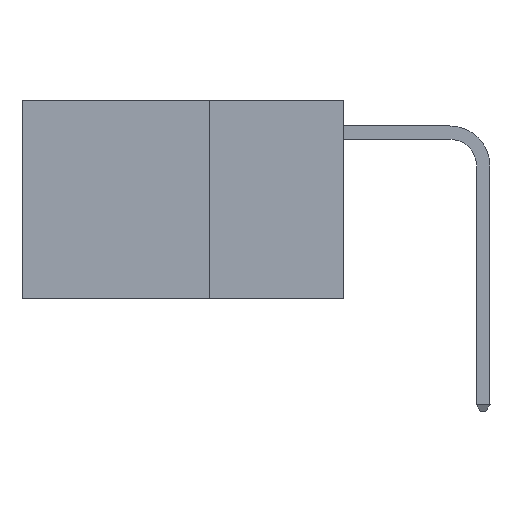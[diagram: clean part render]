
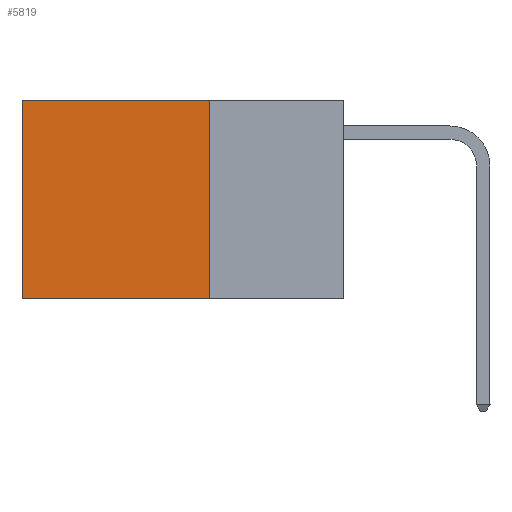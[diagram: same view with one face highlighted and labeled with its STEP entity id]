
A CAD part, left-side view. The second image highlights one B-rep face of the part: STEP entity #5819.
In plain terms, the highlighted planar face has unit normal (-1, 0, 0).
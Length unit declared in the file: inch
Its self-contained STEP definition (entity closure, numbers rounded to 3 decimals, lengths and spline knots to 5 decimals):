
#1422 = DIRECTION ( 'NONE',  ( 0., 0., -1. ) ) ;
#1533 = CARTESIAN_POINT ( 'NONE',  ( 0.2625, 0.25, 0. ) ) ;
#1546 = CARTESIAN_POINT ( 'NONE',  ( 0.2625, 0.6, 0. ) ) ;
#2012 = ORIENTED_EDGE ( 'NONE', *, *, #9931, .F. ) ;
#2030 = VERTEX_POINT ( 'NONE', #15857 ) ;
#3189 = FACE_OUTER_BOUND ( 'NONE', #8906, .T. ) ;
#3850 = VERTEX_POINT ( 'NONE', #1533 ) ;
#4911 = DIRECTION ( 'NONE',  ( 0., 0., -1. ) ) ;
#5016 = CARTESIAN_POINT ( 'NONE',  ( 0.2625, 0.25, 0. ) ) ;
#5265 = DIRECTION ( 'NONE',  ( 0., 1., 0. ) ) ;
#5454 = CARTESIAN_POINT ( 'NONE',  ( 0.2625, 0.25, 0. ) ) ;
#5637 = VECTOR ( 'NONE', #6112, 39.37008 ) ;
#5819 = ADVANCED_FACE ( 'NONE', ( #3189 ), #13883, .F. ) ;
#6083 = LINE ( 'NONE', #1546, #6202 ) ;
#6112 = DIRECTION ( 'NONE',  ( 0., 1., 0. ) ) ;
#6154 = VERTEX_POINT ( 'NONE', #17012 ) ;
#6202 = VECTOR ( 'NONE', #1422, 39.37008 ) ;
#6820 = ORIENTED_EDGE ( 'NONE', *, *, #7748, .T. ) ;
#7059 = ORIENTED_EDGE ( 'NONE', *, *, #8143, .T. ) ;
#7748 = EDGE_CURVE ( 'NONE', #3850, #2030, #8345, .T. ) ;
#7772 = EDGE_CURVE ( 'NONE', #3850, #8298, #8010, .T. ) ;
#7924 = VECTOR ( 'NONE', #4911, 39.37008 ) ;
#7942 = CARTESIAN_POINT ( 'NONE',  ( 0.2625, 0.25, -0.37 ) ) ;
#8010 = LINE ( 'NONE', #5016, #7924 ) ;
#8143 = EDGE_CURVE ( 'NONE', #2030, #6154, #6083, .T. ) ;
#8298 = VERTEX_POINT ( 'NONE', #7942 ) ;
#8345 = LINE ( 'NONE', #5454, #8379 ) ;
#8379 = VECTOR ( 'NONE', #5265, 39.37008 ) ;
#8906 = EDGE_LOOP ( 'NONE', ( #7059, #2012, #17795, #6820 ) ) ;
#9931 = EDGE_CURVE ( 'NONE', #8298, #6154, #12962, .T. ) ;
#12689 = CARTESIAN_POINT ( 'NONE',  ( 0.2625, 0.25, 0. ) ) ;
#12962 = LINE ( 'NONE', #15616, #5637 ) ;
#13620 = AXIS2_PLACEMENT_3D ( 'NONE', #12689, #17352, #17408 ) ;
#13883 = PLANE ( 'NONE',  #13620 ) ;
#15616 = CARTESIAN_POINT ( 'NONE',  ( 0.2625, 0.25, -0.37 ) ) ;
#15857 = CARTESIAN_POINT ( 'NONE',  ( 0.2625, 0.6, 0. ) ) ;
#17012 = CARTESIAN_POINT ( 'NONE',  ( 0.2625, 0.6, -0.37 ) ) ;
#17352 = DIRECTION ( 'NONE',  ( 1., 0., 0. ) ) ;
#17408 = DIRECTION ( 'NONE',  ( 0., 0., -1. ) ) ;
#17795 = ORIENTED_EDGE ( 'NONE', *, *, #7772, .F. ) ;
